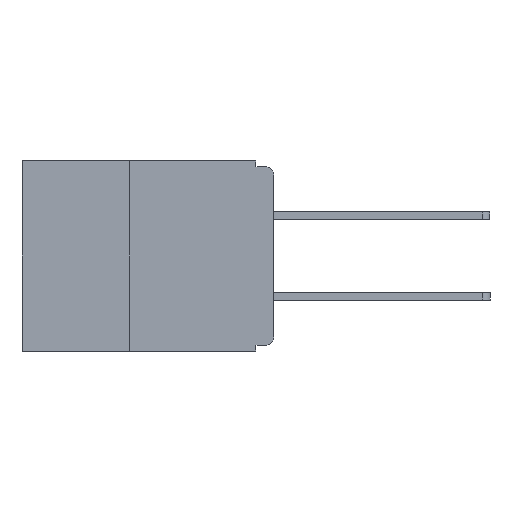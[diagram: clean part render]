
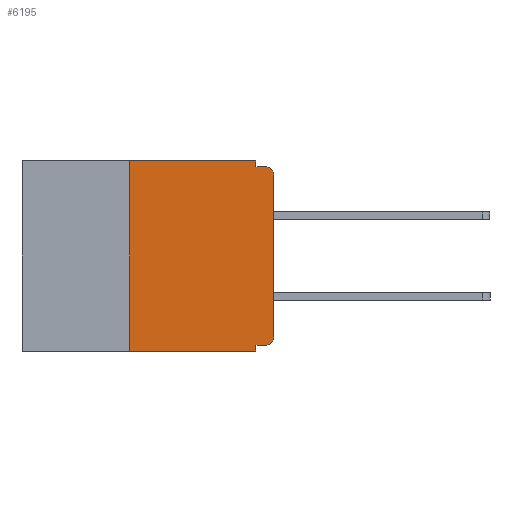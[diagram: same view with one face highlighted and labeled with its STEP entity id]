
A CAD part, left-side view. The second image highlights one B-rep face of the part: STEP entity #6195.
In plain terms, the highlighted planar face has unit normal (-1, 0, 0).
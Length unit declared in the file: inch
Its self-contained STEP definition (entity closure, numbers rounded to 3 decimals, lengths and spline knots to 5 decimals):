
#792 = VERTEX_POINT ( 'NONE', #9031 ) ;
#1231 = ORIENTED_EDGE ( 'NONE', *, *, #19248, .F. ) ;
#1412 = VERTEX_POINT ( 'NONE', #4477 ) ;
#1548 = ORIENTED_EDGE ( 'NONE', *, *, #25318, .F. ) ;
#1785 = VERTEX_POINT ( 'NONE', #19326 ) ;
#2109 = DIRECTION ( 'NONE',  ( 1., 0., 0. ) ) ;
#2204 = ORIENTED_EDGE ( 'NONE', *, *, #14820, .F. ) ;
#2477 = VECTOR ( 'NONE', #25018, 39.37008 ) ;
#2870 = CARTESIAN_POINT ( 'NONE',  ( 0., 0.437, 0. ) ) ;
#3340 = ORIENTED_EDGE ( 'NONE', *, *, #18695, .T. ) ;
#3889 = VECTOR ( 'NONE', #16501, 39.37008 ) ;
#4477 = CARTESIAN_POINT ( 'NONE',  ( 0., 0.031, 0. ) ) ;
#4562 = VECTOR ( 'NONE', #23089, 39.37008 ) ;
#4612 = EDGE_CURVE ( 'NONE', #19147, #792, #9616, .T. ) ;
#4688 = CARTESIAN_POINT ( 'NONE',  ( 0., 0., 0. ) ) ;
#4841 = CARTESIAN_POINT ( 'NONE',  ( 0., 0.015, -0.305 ) ) ;
#5126 = CARTESIAN_POINT ( 'NONE',  ( 0., 0.031, -0.33 ) ) ;
#5570 = CARTESIAN_POINT ( 'NONE',  ( 0., 0.25, -0.33 ) ) ;
#5672 = CIRCLE ( 'NONE', #24254, 0.015 ) ;
#5710 = ORIENTED_EDGE ( 'NONE', *, *, #20204, .F. ) ;
#6195 = ADVANCED_FACE ( 'NONE', ( #26320 ), #17748, .F. ) ;
#6636 = VECTOR ( 'NONE', #25835, 39.37008 ) ;
#6988 = DIRECTION ( 'NONE',  ( 0., 0., -1. ) ) ;
#7130 = VERTEX_POINT ( 'NONE', #13991 ) ;
#7153 = CARTESIAN_POINT ( 'NONE',  ( 0., 0.437, 0. ) ) ;
#7733 = DIRECTION ( 'NONE',  ( 0., 0., 1. ) ) ;
#7809 = DIRECTION ( 'NONE',  ( -1., 0., 0. ) ) ;
#8520 = LINE ( 'NONE', #5570, #18987 ) ;
#8781 = VERTEX_POINT ( 'NONE', #5126 ) ;
#9031 = CARTESIAN_POINT ( 'NONE',  ( 0., 0.031, -0.32 ) ) ;
#9616 = LINE ( 'NONE', #16436, #3889 ) ;
#10015 = CIRCLE ( 'NONE', #21131, 0.015 ) ;
#10099 = EDGE_LOOP ( 'NONE', ( #22551, #25447, #2204, #1548, #1231, #19485, #19170, #5710, #16910, #3340 ) ) ;
#10203 = CARTESIAN_POINT ( 'NONE',  ( 0., 0., -0.305 ) ) ;
#11528 = VECTOR ( 'NONE', #21095, 39.37008 ) ;
#12929 = DIRECTION ( 'NONE',  ( 0., 0., -1. ) ) ;
#13438 = CARTESIAN_POINT ( 'NONE',  ( 0., 0.031, -0.01 ) ) ;
#13991 = CARTESIAN_POINT ( 'NONE',  ( 0., 0.25, 0. ) ) ;
#14757 = DIRECTION ( 'NONE',  ( 0., 0., -1. ) ) ;
#14773 = CARTESIAN_POINT ( 'NONE',  ( 0., 0., -0.01 ) ) ;
#14820 = EDGE_CURVE ( 'NONE', #18108, #19987, #18422, .T. ) ;
#15192 = EDGE_CURVE ( 'NONE', #1785, #7130, #8520, .T. ) ;
#16105 = VECTOR ( 'NONE', #19401, 39.37008 ) ;
#16436 = CARTESIAN_POINT ( 'NONE',  ( 0., 0., -0.32 ) ) ;
#16501 = DIRECTION ( 'NONE',  ( 0., 1., 0. ) ) ;
#16910 = ORIENTED_EDGE ( 'NONE', *, *, #4612, .F. ) ;
#17748 = PLANE ( 'NONE',  #20750 ) ;
#18108 = VERTEX_POINT ( 'NONE', #13438 ) ;
#18308 = CARTESIAN_POINT ( 'NONE',  ( 0., 0.015, -0.01 ) ) ;
#18422 = LINE ( 'NONE', #14773, #11528 ) ;
#18695 = EDGE_CURVE ( 'NONE', #19147, #25819, #10015, .T. ) ;
#18987 = VECTOR ( 'NONE', #7733, 39.37008 ) ;
#18993 = CARTESIAN_POINT ( 'NONE',  ( 0., 0.031, 0. ) ) ;
#19011 = CARTESIAN_POINT ( 'NONE',  ( 0., 0.031, -0.33 ) ) ;
#19147 = VERTEX_POINT ( 'NONE', #25471 ) ;
#19170 = ORIENTED_EDGE ( 'NONE', *, *, #25917, .T. ) ;
#19248 = EDGE_CURVE ( 'NONE', #7130, #1412, #23239, .T. ) ;
#19326 = CARTESIAN_POINT ( 'NONE',  ( 0., 0.25, -0.33 ) ) ;
#19355 = LINE ( 'NONE', #22956, #2477 ) ;
#19401 = DIRECTION ( 'NONE',  ( 0., 0., 1. ) ) ;
#19485 = ORIENTED_EDGE ( 'NONE', *, *, #15192, .F. ) ;
#19545 = DIRECTION ( 'NONE',  ( -1., 0., 0. ) ) ;
#19987 = VERTEX_POINT ( 'NONE', #18308 ) ;
#20204 = EDGE_CURVE ( 'NONE', #792, #8781, #21326, .T. ) ;
#20368 = CARTESIAN_POINT ( 'NONE',  ( 0., 0.015, -0.025 ) ) ;
#20370 = VERTEX_POINT ( 'NONE', #21623 ) ;
#20750 = AXIS2_PLACEMENT_3D ( 'NONE', #2870, #2109, #12929 ) ;
#20984 = LINE ( 'NONE', #4688, #16105 ) ;
#21095 = DIRECTION ( 'NONE',  ( 0., -1., 0. ) ) ;
#21131 = AXIS2_PLACEMENT_3D ( 'NONE', #4841, #19545, #6988 ) ;
#21326 = LINE ( 'NONE', #19011, #4562 ) ;
#21623 = CARTESIAN_POINT ( 'NONE',  ( 0., 0., -0.025 ) ) ;
#22364 = DIRECTION ( 'NONE',  ( 0., 0., -1. ) ) ;
#22551 = ORIENTED_EDGE ( 'NONE', *, *, #26064, .T. ) ;
#22956 = CARTESIAN_POINT ( 'NONE',  ( 0., 0.437, -0.33 ) ) ;
#23089 = DIRECTION ( 'NONE',  ( 0., 0., -1. ) ) ;
#23239 = LINE ( 'NONE', #7153, #6636 ) ;
#23843 = VECTOR ( 'NONE', #14757, 39.37008 ) ;
#23924 = EDGE_CURVE ( 'NONE', #20370, #19987, #5672, .T. ) ;
#24254 = AXIS2_PLACEMENT_3D ( 'NONE', #20368, #7809, #22364 ) ;
#24500 = LINE ( 'NONE', #18993, #23843 ) ;
#25018 = DIRECTION ( 'NONE',  ( 0., -1., 0. ) ) ;
#25318 = EDGE_CURVE ( 'NONE', #1412, #18108, #24500, .T. ) ;
#25447 = ORIENTED_EDGE ( 'NONE', *, *, #23924, .T. ) ;
#25471 = CARTESIAN_POINT ( 'NONE',  ( 0., 0.015, -0.32 ) ) ;
#25819 = VERTEX_POINT ( 'NONE', #10203 ) ;
#25835 = DIRECTION ( 'NONE',  ( 0., -1., 0. ) ) ;
#25917 = EDGE_CURVE ( 'NONE', #1785, #8781, #19355, .T. ) ;
#26064 = EDGE_CURVE ( 'NONE', #25819, #20370, #20984, .T. ) ;
#26320 = FACE_OUTER_BOUND ( 'NONE', #10099, .T. ) ;
